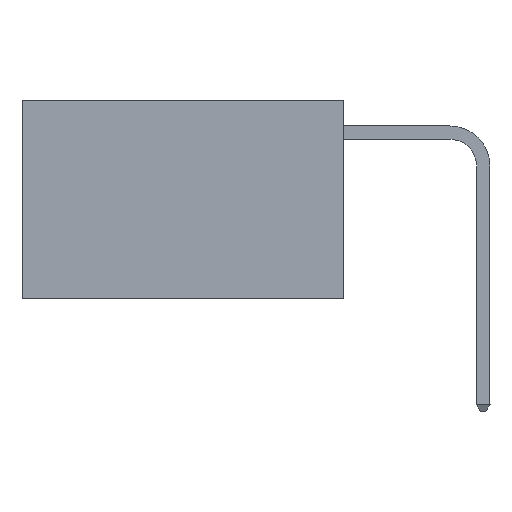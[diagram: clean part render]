
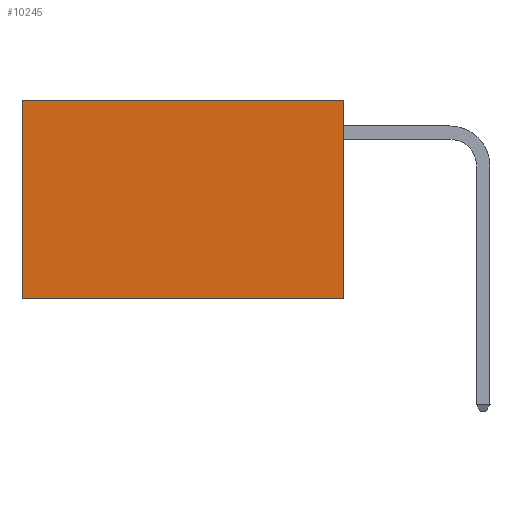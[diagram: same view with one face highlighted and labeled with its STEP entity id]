
A CAD part, left-side view. The second image highlights one B-rep face of the part: STEP entity #10245.
In plain terms, the highlighted planar face has unit normal (-1, 0, 0).
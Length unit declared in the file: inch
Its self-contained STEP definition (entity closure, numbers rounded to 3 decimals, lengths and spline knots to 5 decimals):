
#384 = CARTESIAN_POINT ( 'NONE',  ( 0.2625, 0., -0.37 ) ) ;
#735 = ORIENTED_EDGE ( 'NONE', *, *, #13107, .F. ) ;
#1180 = LINE ( 'NONE', #1452, #10331 ) ;
#1452 = CARTESIAN_POINT ( 'NONE',  ( 0.2625, 0.6, 0. ) ) ;
#1649 = VERTEX_POINT ( 'NONE', #9960 ) ;
#2078 = ORIENTED_EDGE ( 'NONE', *, *, #7262, .T. ) ;
#2967 = EDGE_CURVE ( 'NONE', #4863, #11861, #1180, .T. ) ;
#3182 = VECTOR ( 'NONE', #4595, 39.37008 ) ;
#3442 = ORIENTED_EDGE ( 'NONE', *, *, #11050, .F. ) ;
#3861 = DIRECTION ( 'NONE',  ( 0., 0., -1. ) ) ;
#4595 = DIRECTION ( 'NONE',  ( 0., 1., 0. ) ) ;
#4863 = VERTEX_POINT ( 'NONE', #8668 ) ;
#6167 = DIRECTION ( 'NONE',  ( 0., 0., -1. ) ) ;
#6458 = LINE ( 'NONE', #10098, #9227 ) ;
#6607 = DIRECTION ( 'NONE',  ( 0., 0., -1. ) ) ;
#6747 = LINE ( 'NONE', #7054, #3182 ) ;
#7054 = CARTESIAN_POINT ( 'NONE',  ( 0.2625, 0., -0.37 ) ) ;
#7058 = CARTESIAN_POINT ( 'NONE',  ( 0.2625, 0.6, -0.37 ) ) ;
#7262 = EDGE_CURVE ( 'NONE', #1649, #4863, #11487, .T. ) ;
#7796 = CARTESIAN_POINT ( 'NONE',  ( 0.2625, 0., 0. ) ) ;
#8047 = EDGE_LOOP ( 'NONE', ( #9825, #735, #3442, #2078 ) ) ;
#8377 = CARTESIAN_POINT ( 'NONE',  ( 0.2625, 0., 0. ) ) ;
#8382 = VECTOR ( 'NONE', #10169, 39.37008 ) ;
#8668 = CARTESIAN_POINT ( 'NONE',  ( 0.2625, 0.6, 0. ) ) ;
#8989 = VERTEX_POINT ( 'NONE', #384 ) ;
#9227 = VECTOR ( 'NONE', #6607, 39.37008 ) ;
#9825 = ORIENTED_EDGE ( 'NONE', *, *, #2967, .T. ) ;
#9960 = CARTESIAN_POINT ( 'NONE',  ( 0.2625, 0., 0. ) ) ;
#10098 = CARTESIAN_POINT ( 'NONE',  ( 0.2625, 0., 0. ) ) ;
#10169 = DIRECTION ( 'NONE',  ( 0., 1., 0. ) ) ;
#10245 = ADVANCED_FACE ( 'NONE', ( #12313 ), #12987, .F. ) ;
#10331 = VECTOR ( 'NONE', #6167, 39.37008 ) ;
#10944 = DIRECTION ( 'NONE',  ( 1., 0., 0. ) ) ;
#11050 = EDGE_CURVE ( 'NONE', #1649, #8989, #6458, .T. ) ;
#11425 = AXIS2_PLACEMENT_3D ( 'NONE', #8377, #10944, #3861 ) ;
#11487 = LINE ( 'NONE', #7796, #8382 ) ;
#11861 = VERTEX_POINT ( 'NONE', #7058 ) ;
#12313 = FACE_OUTER_BOUND ( 'NONE', #8047, .T. ) ;
#12987 = PLANE ( 'NONE',  #11425 ) ;
#13107 = EDGE_CURVE ( 'NONE', #8989, #11861, #6747, .T. ) ;
